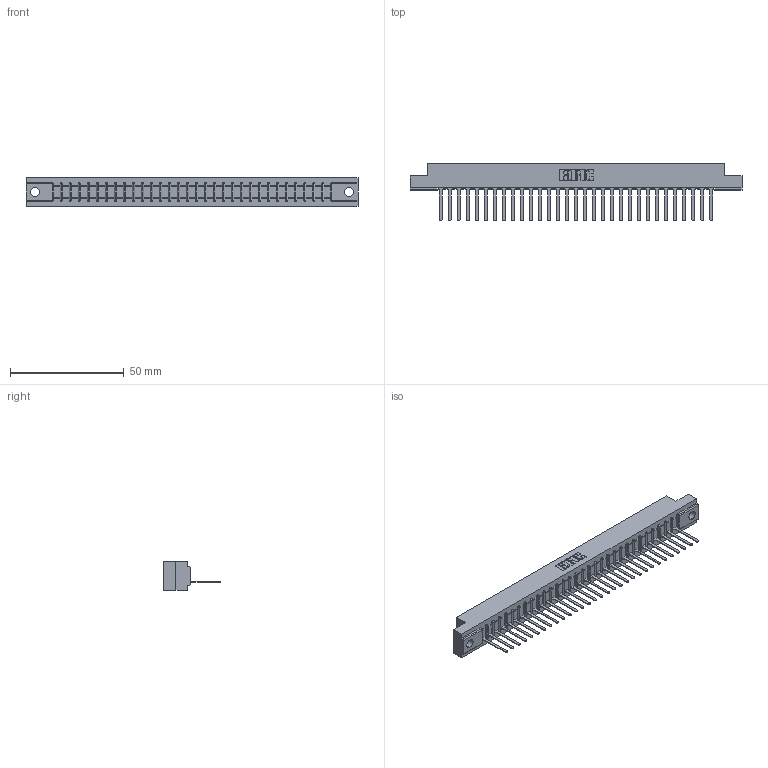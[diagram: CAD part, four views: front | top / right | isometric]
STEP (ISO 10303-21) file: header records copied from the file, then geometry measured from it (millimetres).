
FILE_DESCRIPTION (( 'STEP AP203' ), '1' );
FILE_NAME ('307-031-547-102.STEP', '2019-09-04T00:46:17', ( '' ), ( '' ), 'SwSTEP 2.0', 'SolidWorks 2016', '' );
FILE_SCHEMA (( 'CONFIG_CONTROL_DESIGN' ));
Length unit declared in the file: inch
Products named in the file (3): 307-031-547-102; 307 Part_.128 Dia Mounting Holes; 307-290-001_547
Assembly tree (32 placements, depth 2):
  307-031-547-102
    307 Part_.128 Dia Mounting Holes
    307-290-001_547  x31
Bounding box: 145.85 x 25.43 x 12.7 mm (x, y, z)
Volume: 15061.7 mm3; surface area: 16058.9 mm2
Topology: 32 solids, 32 shells, 1886 faces, 5345 edges, 3434 vertices
Faces by surface type: plane 1217, cylinder 605, sphere 64
Entity records: 27902 total; most frequent: CARTESIAN_POINT 4696, ORIENTED_EDGE 4682, DIRECTION 4573, EDGE_CURVE 2341, VECTOR 1791, LINE 1791, VERTEX_POINT 1514, AXIS2_PLACEMENT_3D 1391
